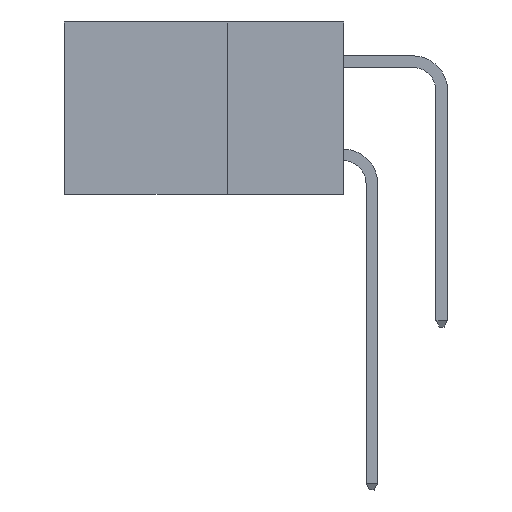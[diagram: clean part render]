
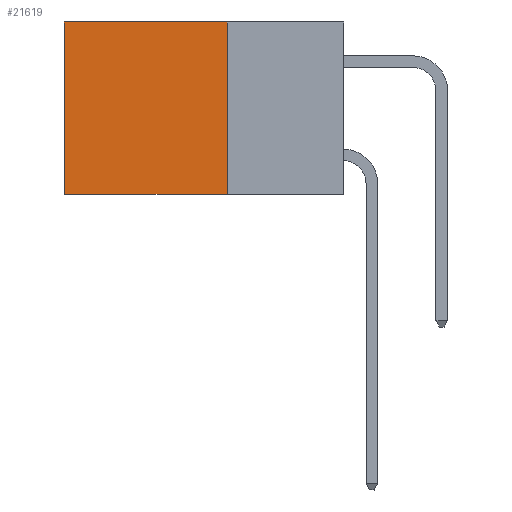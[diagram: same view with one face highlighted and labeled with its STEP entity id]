
A CAD part, left-side view. The second image highlights one B-rep face of the part: STEP entity #21619.
In plain terms, the highlighted planar face has unit normal (-1, 0, 0).
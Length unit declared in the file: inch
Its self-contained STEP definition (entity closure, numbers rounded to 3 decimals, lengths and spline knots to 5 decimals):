
#206 = CARTESIAN_POINT ( 'NONE',  ( 0.298, 0.6, 0. ) ) ;
#287 = EDGE_CURVE ( 'NONE', #30647, #1991, #4916, .T. ) ;
#542 = EDGE_LOOP ( 'NONE', ( #12320, #15834, #21773, #18114 ) ) ;
#991 = LINE ( 'NONE', #25086, #6727 ) ;
#1991 = VERTEX_POINT ( 'NONE', #206 ) ;
#2765 = VERTEX_POINT ( 'NONE', #9083 ) ;
#3101 = FACE_OUTER_BOUND ( 'NONE', #542, .T. ) ;
#4469 = CARTESIAN_POINT ( 'NONE',  ( 0.298, 0.25, 0. ) ) ;
#4491 = VECTOR ( 'NONE', #8450, 39.37008 ) ;
#4916 = LINE ( 'NONE', #27452, #17717 ) ;
#6727 = VECTOR ( 'NONE', #27493, 39.37008 ) ;
#8063 = DIRECTION ( 'NONE',  ( 0., 1., 0. ) ) ;
#8112 = EDGE_CURVE ( 'NONE', #30647, #27685, #991, .T. ) ;
#8450 = DIRECTION ( 'NONE',  ( 0., 0., -1. ) ) ;
#9083 = CARTESIAN_POINT ( 'NONE',  ( 0.298, 0.6, -0.37 ) ) ;
#9313 = DIRECTION ( 'NONE',  ( 0., 0., -1. ) ) ;
#9551 = DIRECTION ( 'NONE',  ( 0., 1., 0. ) ) ;
#9636 = VECTOR ( 'NONE', #8063, 39.37008 ) ;
#12320 = ORIENTED_EDGE ( 'NONE', *, *, #23289, .T. ) ;
#14991 = CARTESIAN_POINT ( 'NONE',  ( 0.298, 0.25, -0.37 ) ) ;
#15834 = ORIENTED_EDGE ( 'NONE', *, *, #15873, .F. ) ;
#15873 = EDGE_CURVE ( 'NONE', #27685, #2765, #30263, .T. ) ;
#17294 = LINE ( 'NONE', #27623, #4491 ) ;
#17717 = VECTOR ( 'NONE', #9551, 39.37008 ) ;
#18114 = ORIENTED_EDGE ( 'NONE', *, *, #287, .T. ) ;
#21252 = PLANE ( 'NONE',  #21655 ) ;
#21619 = ADVANCED_FACE ( 'NONE', ( #3101 ), #21252, .F. ) ;
#21655 = AXIS2_PLACEMENT_3D ( 'NONE', #4469, #23665, #9313 ) ;
#21773 = ORIENTED_EDGE ( 'NONE', *, *, #8112, .F. ) ;
#23289 = EDGE_CURVE ( 'NONE', #1991, #2765, #17294, .T. ) ;
#23665 = DIRECTION ( 'NONE',  ( 1., 0., 0. ) ) ;
#25086 = CARTESIAN_POINT ( 'NONE',  ( 0.298, 0.25, 0. ) ) ;
#27245 = CARTESIAN_POINT ( 'NONE',  ( 0.298, 0.25, -0.37 ) ) ;
#27452 = CARTESIAN_POINT ( 'NONE',  ( 0.298, 0.25, 0. ) ) ;
#27493 = DIRECTION ( 'NONE',  ( 0., 0., -1. ) ) ;
#27623 = CARTESIAN_POINT ( 'NONE',  ( 0.298, 0.6, 0. ) ) ;
#27685 = VERTEX_POINT ( 'NONE', #14991 ) ;
#28643 = CARTESIAN_POINT ( 'NONE',  ( 0.298, 0.25, 0. ) ) ;
#30263 = LINE ( 'NONE', #27245, #9636 ) ;
#30647 = VERTEX_POINT ( 'NONE', #28643 ) ;
